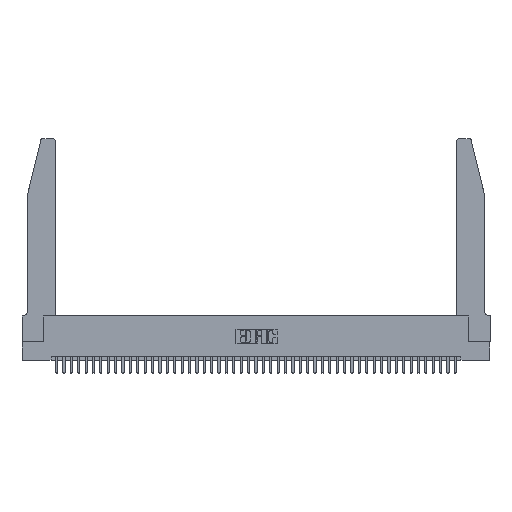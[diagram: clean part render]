
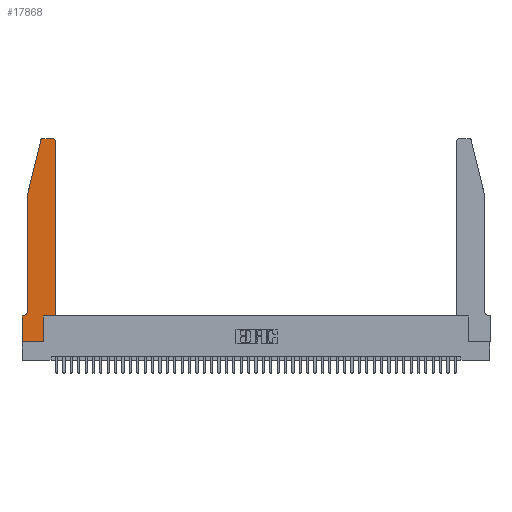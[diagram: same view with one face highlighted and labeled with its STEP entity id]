
A CAD part, top view. The second image highlights one B-rep face of the part: STEP entity #17868.
In plain terms, the highlighted planar face has unit normal (0, 0, 1).
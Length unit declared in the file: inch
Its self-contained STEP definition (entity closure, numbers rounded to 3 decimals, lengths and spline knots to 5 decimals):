
#838 = VECTOR ( 'NONE', #8744, 39.37008 ) ;
#1493 = EDGE_CURVE ( 'NONE', #27455, #12569, #35157, .T. ) ;
#2255 = VERTEX_POINT ( 'NONE', #44582 ) ;
#2262 = LINE ( 'NONE', #45011, #41997 ) ;
#2667 = VECTOR ( 'NONE', #45986, 39.37008 ) ;
#3363 = EDGE_CURVE ( 'NONE', #2255, #36950, #36153, .T. ) ;
#4091 = CARTESIAN_POINT ( 'NONE',  ( 0., 0.35, 0.37 ) ) ;
#5719 = ORIENTED_EDGE ( 'NONE', *, *, #27748, .T. ) ;
#6271 = EDGE_CURVE ( 'NONE', #12569, #13124, #19529, .T. ) ;
#6932 = VERTEX_POINT ( 'NONE', #36598 ) ;
#7348 = CARTESIAN_POINT ( 'NONE',  ( 0.4505, 0.35, 0.37 ) ) ;
#8069 = AXIS2_PLACEMENT_3D ( 'NONE', #39734, #10772, #14383 ) ;
#8283 = DIRECTION ( 'NONE',  ( 0., -1., 0. ) ) ;
#8722 = CARTESIAN_POINT ( 'NONE',  ( 0.0755, 2., 0.37 ) ) ;
#8744 = DIRECTION ( 'NONE',  ( 0., -1., 0. ) ) ;
#9381 = CARTESIAN_POINT ( 'NONE',  ( 0.2865, 0.35, 0.37 ) ) ;
#9907 = ORIENTED_EDGE ( 'NONE', *, *, #6271, .T. ) ;
#10663 = FACE_OUTER_BOUND ( 'NONE', #27833, .T. ) ;
#10772 = DIRECTION ( 'NONE',  ( 0., 0., -1. ) ) ;
#10996 = ORIENTED_EDGE ( 'NONE', *, *, #41922, .T. ) ;
#11204 = ORIENTED_EDGE ( 'NONE', *, *, #40598, .T. ) ;
#12239 = CARTESIAN_POINT ( 'NONE',  ( 0.284, 2.72, 0.37 ) ) ;
#12569 = VERTEX_POINT ( 'NONE', #32743 ) ;
#12892 = EDGE_CURVE ( 'NONE', #40597, #27552, #38575, .T. ) ;
#13124 = VERTEX_POINT ( 'NONE', #40798 ) ;
#13846 = VERTEX_POINT ( 'NONE', #44038 ) ;
#14206 = CIRCLE ( 'NONE', #8069, 0.07 ) ;
#14383 = DIRECTION ( 'NONE',  ( -1., 0., 0. ) ) ;
#15113 = LINE ( 'NONE', #18168, #42034 ) ;
#15727 = CARTESIAN_POINT ( 'NONE',  ( 0.0755, 0.35, 0.37 ) ) ;
#16678 = VECTOR ( 'NONE', #28203, 39.37008 ) ;
#16738 = ORIENTED_EDGE ( 'NONE', *, *, #25351, .T. ) ;
#17240 = LINE ( 'NONE', #8722, #17826 ) ;
#17401 = DIRECTION ( 'NONE',  ( -0.239, -0.971, 0. ) ) ;
#17826 = VECTOR ( 'NONE', #8283, 39.37008 ) ;
#17868 = ADVANCED_FACE ( 'NONE', ( #10663 ), #24865, .T. ) ;
#18046 = ORIENTED_EDGE ( 'NONE', *, *, #39456, .T. ) ;
#18168 = CARTESIAN_POINT ( 'NONE',  ( 0.2865, 0.35, 0.37 ) ) ;
#19271 = VERTEX_POINT ( 'NONE', #40947 ) ;
#19471 = ORIENTED_EDGE ( 'NONE', *, *, #1493, .T. ) ;
#19529 = LINE ( 'NONE', #7348, #29079 ) ;
#20522 = CARTESIAN_POINT ( 'NONE',  ( 0.0755, 2., 0.37 ) ) ;
#20998 = CARTESIAN_POINT ( 'NONE',  ( 0., 0., 0.37 ) ) ;
#23264 = ORIENTED_EDGE ( 'NONE', *, *, #3363, .T. ) ;
#24114 = EDGE_CURVE ( 'NONE', #13124, #13846, #34106, .T. ) ;
#24245 = DIRECTION ( 'NONE',  ( 0., 0., 1. ) ) ;
#24523 = CIRCLE ( 'NONE', #31047, 0.03 ) ;
#24865 = PLANE ( 'NONE',  #24977 ) ;
#24977 = AXIS2_PLACEMENT_3D ( 'NONE', #28296, #24245, #35492 ) ;
#25351 = EDGE_CURVE ( 'NONE', #19271, #6932, #24523, .T. ) ;
#25388 = VERTEX_POINT ( 'NONE', #44644 ) ;
#27455 = VERTEX_POINT ( 'NONE', #9381 ) ;
#27552 = VERTEX_POINT ( 'NONE', #31804 ) ;
#27748 = EDGE_CURVE ( 'NONE', #25388, #2255, #14206, .T. ) ;
#27833 = EDGE_LOOP ( 'NONE', ( #18046, #16738, #29060, #11204, #5719, #23264, #10996, #29781, #36245, #19471, #9907, #40890 ) ) ;
#28203 = DIRECTION ( 'NONE',  ( 1., 0., 0. ) ) ;
#28296 = CARTESIAN_POINT ( 'NONE',  ( 0., 0.35, 0.37 ) ) ;
#29060 = ORIENTED_EDGE ( 'NONE', *, *, #34911, .T. ) ;
#29079 = VECTOR ( 'NONE', #32397, 39.37008 ) ;
#29282 = AXIS2_PLACEMENT_3D ( 'NONE', #35455, #35296, #31709 ) ;
#29781 = ORIENTED_EDGE ( 'NONE', *, *, #12892, .T. ) ;
#31047 = AXIS2_PLACEMENT_3D ( 'NONE', #12239, #37460, #44489 ) ;
#31229 = CARTESIAN_POINT ( 'NONE',  ( 0.0755, 2., 0.37 ) ) ;
#31499 = CARTESIAN_POINT ( 'NONE',  ( 0.4505, 0.35, 0.37 ) ) ;
#31709 = DIRECTION ( 'NONE',  ( 1., 0., 0. ) ) ;
#31804 = CARTESIAN_POINT ( 'NONE',  ( 0.2865, 0., 0.37 ) ) ;
#32397 = DIRECTION ( 'NONE',  ( 0., 1., 0. ) ) ;
#32743 = CARTESIAN_POINT ( 'NONE',  ( 0.4505, 0.35, 0.37 ) ) ;
#33721 = EDGE_CURVE ( 'NONE', #27552, #27455, #15113, .T. ) ;
#34073 = DIRECTION ( 'NONE',  ( -1., 0., 0. ) ) ;
#34106 = CIRCLE ( 'NONE', #29282, 0.03 ) ;
#34422 = LINE ( 'NONE', #31229, #36086 ) ;
#34443 = LINE ( 'NONE', #36957, #838 ) ;
#34549 = DIRECTION ( 'NONE',  ( -1., 0., 0. ) ) ;
#34911 = EDGE_CURVE ( 'NONE', #6932, #39031, #34422, .T. ) ;
#35157 = LINE ( 'NONE', #31499, #2667 ) ;
#35296 = DIRECTION ( 'NONE',  ( 0., 0., 1. ) ) ;
#35455 = CARTESIAN_POINT ( 'NONE',  ( 0.4205, 2.72, 0.37 ) ) ;
#35492 = DIRECTION ( 'NONE',  ( 1., 0., 0. ) ) ;
#36053 = DIRECTION ( 'NONE',  ( 0., 1., 0. ) ) ;
#36086 = VECTOR ( 'NONE', #17401, 39.37008 ) ;
#36153 = LINE ( 'NONE', #15727, #37268 ) ;
#36245 = ORIENTED_EDGE ( 'NONE', *, *, #33721, .T. ) ;
#36598 = CARTESIAN_POINT ( 'NONE',  ( 0.25487, 2.72718, 0.37 ) ) ;
#36928 = CARTESIAN_POINT ( 'NONE',  ( 0., 0., 0.37 ) ) ;
#36950 = VERTEX_POINT ( 'NONE', #4091 ) ;
#36957 = CARTESIAN_POINT ( 'NONE',  ( 0., 0., 0.37 ) ) ;
#37268 = VECTOR ( 'NONE', #34073, 39.37008 ) ;
#37460 = DIRECTION ( 'NONE',  ( 0., 0., 1. ) ) ;
#38575 = LINE ( 'NONE', #20998, #16678 ) ;
#39031 = VERTEX_POINT ( 'NONE', #20522 ) ;
#39456 = EDGE_CURVE ( 'NONE', #13846, #19271, #2262, .T. ) ;
#39734 = CARTESIAN_POINT ( 'NONE',  ( 0.0055, 0.42, 0.37 ) ) ;
#40597 = VERTEX_POINT ( 'NONE', #36928 ) ;
#40598 = EDGE_CURVE ( 'NONE', #39031, #25388, #17240, .T. ) ;
#40798 = CARTESIAN_POINT ( 'NONE',  ( 0.4505, 2.72, 0.37 ) ) ;
#40890 = ORIENTED_EDGE ( 'NONE', *, *, #24114, .T. ) ;
#40947 = CARTESIAN_POINT ( 'NONE',  ( 0.284, 2.75, 0.37 ) ) ;
#41922 = EDGE_CURVE ( 'NONE', #36950, #40597, #34443, .T. ) ;
#41997 = VECTOR ( 'NONE', #34549, 39.37008 ) ;
#42034 = VECTOR ( 'NONE', #36053, 39.37008 ) ;
#44038 = CARTESIAN_POINT ( 'NONE',  ( 0.4205, 2.75, 0.37 ) ) ;
#44489 = DIRECTION ( 'NONE',  ( 1., 0., 0. ) ) ;
#44582 = CARTESIAN_POINT ( 'NONE',  ( 0.0055, 0.35, 0.37 ) ) ;
#44644 = CARTESIAN_POINT ( 'NONE',  ( 0.0755, 0.42, 0.37 ) ) ;
#45011 = CARTESIAN_POINT ( 'NONE',  ( 0.2605, 2.75, 0.37 ) ) ;
#45986 = DIRECTION ( 'NONE',  ( 1., 0., 0. ) ) ;
